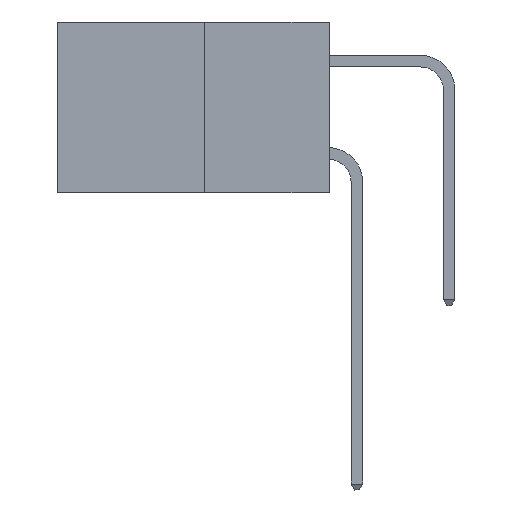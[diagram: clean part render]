
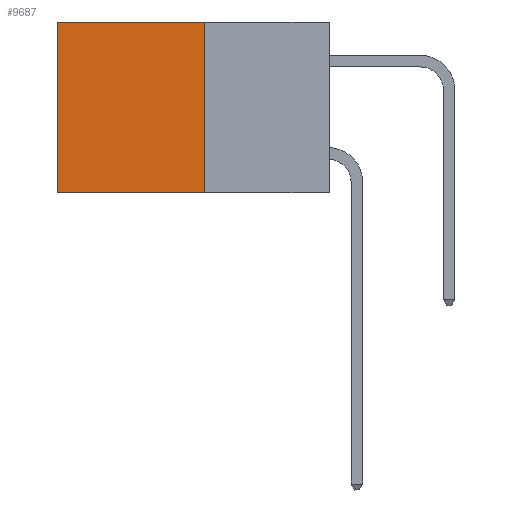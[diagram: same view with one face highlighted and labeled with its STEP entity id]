
A CAD part, left-side view. The second image highlights one B-rep face of the part: STEP entity #9687.
In plain terms, the highlighted planar face has unit normal (-1, 0, 0).
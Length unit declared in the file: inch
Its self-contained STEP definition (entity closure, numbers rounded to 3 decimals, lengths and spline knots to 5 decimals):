
#66 = DIRECTION ( 'NONE',  ( 0., 1., 0. ) ) ;
#263 = CARTESIAN_POINT ( 'NONE',  ( 0.277, 0.59, -0.37 ) ) ;
#1091 = EDGE_CURVE ( 'NONE', #7032, #1126, #8032, .T. ) ;
#1126 = VERTEX_POINT ( 'NONE', #19029 ) ;
#1264 = DIRECTION ( 'NONE',  ( 1., 0., 0. ) ) ;
#1345 = VECTOR ( 'NONE', #16827, 39.37008 ) ;
#1871 = LINE ( 'NONE', #263, #1345 ) ;
#2311 = CARTESIAN_POINT ( 'NONE',  ( 0.277, 0.27, -0.37 ) ) ;
#2446 = DIRECTION ( 'NONE',  ( 0., 0., -1. ) ) ;
#2527 = CARTESIAN_POINT ( 'NONE',  ( 0.277, 0.27, 0. ) ) ;
#3333 = VECTOR ( 'NONE', #12717, 39.37008 ) ;
#4180 = CARTESIAN_POINT ( 'NONE',  ( 0.277, 0.59, -0.37 ) ) ;
#4250 = EDGE_CURVE ( 'NONE', #7032, #7895, #21019, .T. ) ;
#4643 = DIRECTION ( 'NONE',  ( 0., 1., 0. ) ) ;
#4695 = AXIS2_PLACEMENT_3D ( 'NONE', #2311, #1264, #2446 ) ;
#5146 = CARTESIAN_POINT ( 'NONE',  ( 0.277, 0.27, 0. ) ) ;
#7032 = VERTEX_POINT ( 'NONE', #5146 ) ;
#7177 = EDGE_CURVE ( 'NONE', #7895, #7956, #20109, .T. ) ;
#7895 = VERTEX_POINT ( 'NONE', #18321 ) ;
#7956 = VERTEX_POINT ( 'NONE', #4180 ) ;
#8032 = LINE ( 'NONE', #2527, #16183 ) ;
#8605 = EDGE_CURVE ( 'NONE', #1126, #7956, #1871, .T. ) ;
#9687 = ADVANCED_FACE ( 'NONE', ( #14808 ), #20031, .F. ) ;
#9862 = EDGE_LOOP ( 'NONE', ( #13265, #20688, #12782, #20088 ) ) ;
#12717 = DIRECTION ( 'NONE',  ( 0., 0., -1. ) ) ;
#12782 = ORIENTED_EDGE ( 'NONE', *, *, #4250, .F. ) ;
#13265 = ORIENTED_EDGE ( 'NONE', *, *, #8605, .T. ) ;
#14227 = CARTESIAN_POINT ( 'NONE',  ( 0.277, 0.27, -0.37 ) ) ;
#14808 = FACE_OUTER_BOUND ( 'NONE', #9862, .T. ) ;
#16183 = VECTOR ( 'NONE', #4643, 39.37008 ) ;
#16827 = DIRECTION ( 'NONE',  ( 0., 0., -1. ) ) ;
#18321 = CARTESIAN_POINT ( 'NONE',  ( 0.277, 0.27, -0.37 ) ) ;
#19029 = CARTESIAN_POINT ( 'NONE',  ( 0.277, 0.59, 0. ) ) ;
#19594 = VECTOR ( 'NONE', #66, 39.37008 ) ;
#20031 = PLANE ( 'NONE',  #4695 ) ;
#20088 = ORIENTED_EDGE ( 'NONE', *, *, #1091, .T. ) ;
#20109 = LINE ( 'NONE', #14227, #19594 ) ;
#20688 = ORIENTED_EDGE ( 'NONE', *, *, #7177, .F. ) ;
#21019 = LINE ( 'NONE', #21206, #3333 ) ;
#21206 = CARTESIAN_POINT ( 'NONE',  ( 0.277, 0.27, -0.37 ) ) ;
